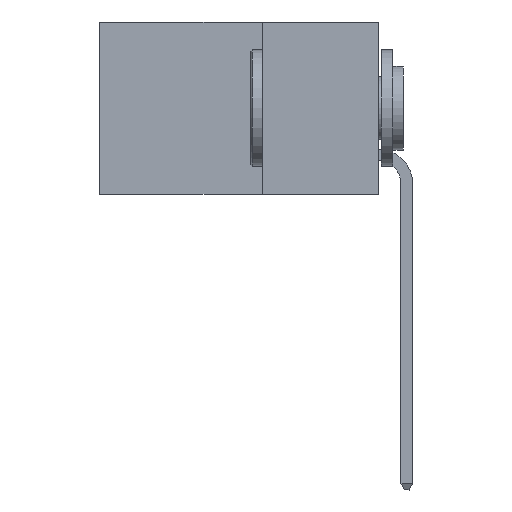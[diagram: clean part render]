
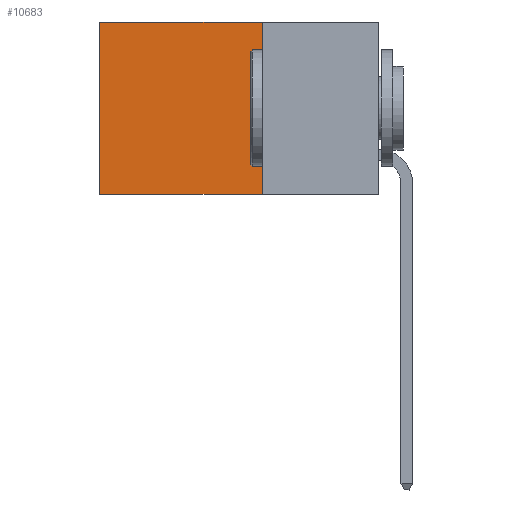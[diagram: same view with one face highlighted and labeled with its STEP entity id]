
A CAD part, left-side view. The second image highlights one B-rep face of the part: STEP entity #10683.
In plain terms, the highlighted planar face has unit normal (-1, 0, 0).
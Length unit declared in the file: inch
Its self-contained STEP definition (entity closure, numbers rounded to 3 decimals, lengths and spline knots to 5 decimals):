
#502 = EDGE_CURVE ( 'NONE', #4859, #27706, #26071, .T. ) ;
#4171 = EDGE_CURVE ( 'NONE', #17014, #27706, #24451, .T. ) ;
#4504 = VECTOR ( 'NONE', #10691, 39.37008 ) ;
#4859 = VERTEX_POINT ( 'NONE', #13194 ) ;
#6671 = EDGE_CURVE ( 'NONE', #7159, #4859, #18402, .T. ) ;
#7159 = VERTEX_POINT ( 'NONE', #15481 ) ;
#10516 = DIRECTION ( 'NONE',  ( 0., 1., 0. ) ) ;
#10683 = ADVANCED_FACE ( 'NONE', ( #31834 ), #11796, .F. ) ;
#10691 = DIRECTION ( 'NONE',  ( 0., 0., -1. ) ) ;
#10815 = VECTOR ( 'NONE', #19544, 39.37008 ) ;
#11017 = ORIENTED_EDGE ( 'NONE', *, *, #502, .F. ) ;
#11031 = CARTESIAN_POINT ( 'NONE',  ( 0.298, 0.25, 0. ) ) ;
#11226 = VECTOR ( 'NONE', #19163, 39.37008 ) ;
#11629 = CARTESIAN_POINT ( 'NONE',  ( 0.298, 0.6, -0.37 ) ) ;
#11796 = PLANE ( 'NONE',  #19937 ) ;
#13194 = CARTESIAN_POINT ( 'NONE',  ( 0.298, 0.25, -0.37 ) ) ;
#14110 = CARTESIAN_POINT ( 'NONE',  ( 0.298, 0.25, -0.37 ) ) ;
#14292 = CARTESIAN_POINT ( 'NONE',  ( 0.298, 0.25, 0. ) ) ;
#15481 = CARTESIAN_POINT ( 'NONE',  ( 0.298, 0.25, 0. ) ) ;
#15812 = ORIENTED_EDGE ( 'NONE', *, *, #6671, .F. ) ;
#16783 = DIRECTION ( 'NONE',  ( 0., 0., -1. ) ) ;
#17014 = VERTEX_POINT ( 'NONE', #20867 ) ;
#18402 = LINE ( 'NONE', #11031, #4504 ) ;
#19163 = DIRECTION ( 'NONE',  ( 0., 0., -1. ) ) ;
#19474 = VECTOR ( 'NONE', #10516, 39.37008 ) ;
#19544 = DIRECTION ( 'NONE',  ( 0., 1., 0. ) ) ;
#19937 = AXIS2_PLACEMENT_3D ( 'NONE', #14292, #31493, #16783 ) ;
#20867 = CARTESIAN_POINT ( 'NONE',  ( 0.298, 0.6, 0. ) ) ;
#22362 = EDGE_LOOP ( 'NONE', ( #23991, #11017, #15812, #24124 ) ) ;
#23991 = ORIENTED_EDGE ( 'NONE', *, *, #4171, .T. ) ;
#24033 = LINE ( 'NONE', #27016, #10815 ) ;
#24124 = ORIENTED_EDGE ( 'NONE', *, *, #24905, .T. ) ;
#24150 = CARTESIAN_POINT ( 'NONE',  ( 0.298, 0.6, 0. ) ) ;
#24451 = LINE ( 'NONE', #24150, #11226 ) ;
#24905 = EDGE_CURVE ( 'NONE', #7159, #17014, #24033, .T. ) ;
#26071 = LINE ( 'NONE', #14110, #19474 ) ;
#27016 = CARTESIAN_POINT ( 'NONE',  ( 0.298, 0.25, 0. ) ) ;
#27706 = VERTEX_POINT ( 'NONE', #11629 ) ;
#31493 = DIRECTION ( 'NONE',  ( 1., 0., 0. ) ) ;
#31834 = FACE_OUTER_BOUND ( 'NONE', #22362, .T. ) ;
